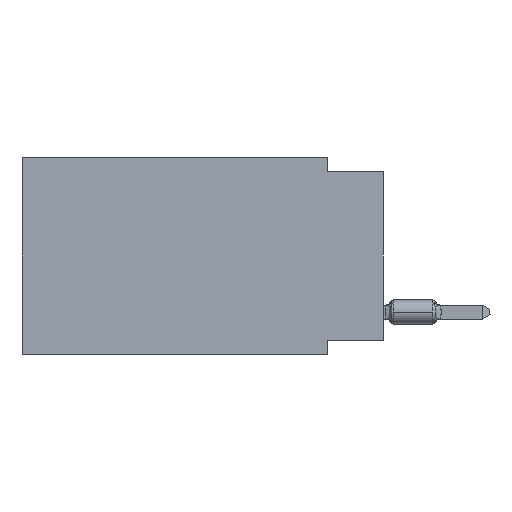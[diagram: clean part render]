
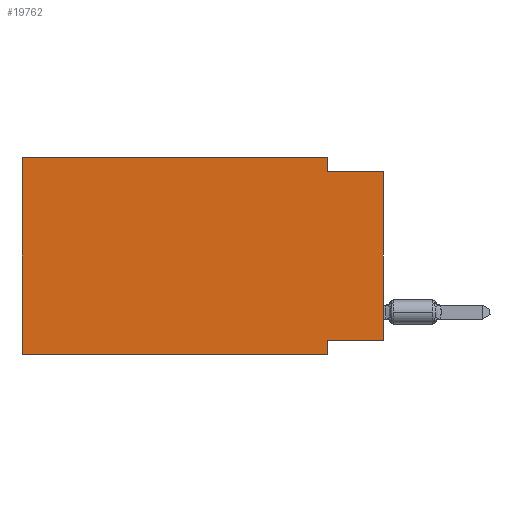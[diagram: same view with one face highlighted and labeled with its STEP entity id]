
A CAD part, left-side view. The second image highlights one B-rep face of the part: STEP entity #19762.
In plain terms, the highlighted planar face has unit normal (-1, 0, 0).
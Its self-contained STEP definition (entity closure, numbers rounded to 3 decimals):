
#37 = EDGE_CURVE ( 'NONE', #6962, #99822, #56680, .T. ) ;
#1829 = EDGE_CURVE ( 'NONE', #4040, #88119, #16245, .T. ) ;
#4040 = VERTEX_POINT ( 'NONE', #28221 ) ;
#5205 = CARTESIAN_POINT ( 'NONE',  ( 0., 0., -0.635 ) ) ;
#6962 = VERTEX_POINT ( 'NONE', #52230 ) ;
#16245 = LINE ( 'NONE', #67094, #36881 ) ;
#16502 = ORIENTED_EDGE ( 'NONE', *, *, #37, .F. ) ;
#18574 = VECTOR ( 'NONE', #83175, 1000. ) ;
#18762 = CARTESIAN_POINT ( 'NONE',  ( 0., 16.383, 0. ) ) ;
#19762 = ADVANCED_FACE ( 'NONE', ( #98889 ), #105676, .F. ) ;
#21310 = VECTOR ( 'NONE', #98407, 1000. ) ;
#28221 = CARTESIAN_POINT ( 'NONE',  ( 0., 16.383, -8.89 ) ) ;
#31546 = AXIS2_PLACEMENT_3D ( 'NONE', #55934, #38963, #63288 ) ;
#32537 = LINE ( 'NONE', #107725, #70098 ) ;
#34352 = CARTESIAN_POINT ( 'NONE',  ( 0., 0., -0.635 ) ) ;
#35883 = CARTESIAN_POINT ( 'NONE',  ( 0., 16.383, 0. ) ) ;
#36881 = VECTOR ( 'NONE', #58614, 1000. ) ;
#37529 = CARTESIAN_POINT ( 'NONE',  ( 0., 0., -8.255 ) ) ;
#38066 = EDGE_LOOP ( 'NONE', ( #58381, #95576, #74974, #60389, #82008, #105151, #45920, #16502 ) ) ;
#38711 = EDGE_CURVE ( 'NONE', #99822, #88119, #32537, .T. ) ;
#38963 = DIRECTION ( 'NONE',  ( 1., 0., 0. ) ) ;
#45920 = ORIENTED_EDGE ( 'NONE', *, *, #38711, .F. ) ;
#47256 = VECTOR ( 'NONE', #78206, 1000. ) ;
#47416 = EDGE_CURVE ( 'NONE', #100924, #77672, #78816, .T. ) ;
#48139 = VERTEX_POINT ( 'NONE', #34352 ) ;
#52230 = CARTESIAN_POINT ( 'NONE',  ( 0., 0., -8.255 ) ) ;
#52786 = CARTESIAN_POINT ( 'NONE',  ( 0., 2.54, 0. ) ) ;
#53641 = CARTESIAN_POINT ( 'NONE',  ( 0., 2.54, -8.89 ) ) ;
#55934 = CARTESIAN_POINT ( 'NONE',  ( 0., 16.383, 0. ) ) ;
#56680 = LINE ( 'NONE', #37529, #88743 ) ;
#58381 = ORIENTED_EDGE ( 'NONE', *, *, #100848, .T. ) ;
#58614 = DIRECTION ( 'NONE',  ( 0., -1., 0. ) ) ;
#58934 = CARTESIAN_POINT ( 'NONE',  ( 0., 0., 0. ) ) ;
#60389 = ORIENTED_EDGE ( 'NONE', *, *, #47416, .F. ) ;
#63288 = DIRECTION ( 'NONE',  ( 0., 0., -1. ) ) ;
#63459 = VECTOR ( 'NONE', #92849, 1000. ) ;
#67094 = CARTESIAN_POINT ( 'NONE',  ( 0., 16.383, -8.89 ) ) ;
#68163 = CARTESIAN_POINT ( 'NONE',  ( 0., 2.54, 0. ) ) ;
#70098 = VECTOR ( 'NONE', #91898, 1000. ) ;
#73494 = CARTESIAN_POINT ( 'NONE',  ( 0., 2.54, -0.635 ) ) ;
#73655 = DIRECTION ( 'NONE',  ( 0., 1., 0. ) ) ;
#74141 = LINE ( 'NONE', #5205, #18574 ) ;
#74974 = ORIENTED_EDGE ( 'NONE', *, *, #99426, .F. ) ;
#77672 = VERTEX_POINT ( 'NONE', #68163 ) ;
#78206 = DIRECTION ( 'NONE',  ( 0., 0., -1. ) ) ;
#78816 = LINE ( 'NONE', #35883, #100861 ) ;
#82008 = ORIENTED_EDGE ( 'NONE', *, *, #94999, .F. ) ;
#82711 = LINE ( 'NONE', #58934, #63459 ) ;
#83175 = DIRECTION ( 'NONE',  ( 0., -1., 0. ) ) ;
#87913 = VERTEX_POINT ( 'NONE', #73494 ) ;
#88119 = VERTEX_POINT ( 'NONE', #53641 ) ;
#88265 = CARTESIAN_POINT ( 'NONE',  ( 0., 2.54, -8.255 ) ) ;
#88743 = VECTOR ( 'NONE', #73655, 1000. ) ;
#91898 = DIRECTION ( 'NONE',  ( 0., 0., -1. ) ) ;
#92849 = DIRECTION ( 'NONE',  ( 0., 0., 1. ) ) ;
#94999 = EDGE_CURVE ( 'NONE', #4040, #100924, #96190, .T. ) ;
#95576 = ORIENTED_EDGE ( 'NONE', *, *, #108126, .F. ) ;
#96190 = LINE ( 'NONE', #18762, #21310 ) ;
#96304 = LINE ( 'NONE', #52786, #47256 ) ;
#98407 = DIRECTION ( 'NONE',  ( 0., 0., 1. ) ) ;
#98889 = FACE_OUTER_BOUND ( 'NONE', #38066, .T. ) ;
#99426 = EDGE_CURVE ( 'NONE', #77672, #87913, #96304, .T. ) ;
#99822 = VERTEX_POINT ( 'NONE', #88265 ) ;
#100848 = EDGE_CURVE ( 'NONE', #6962, #48139, #82711, .T. ) ;
#100861 = VECTOR ( 'NONE', #104805, 1000. ) ;
#100924 = VERTEX_POINT ( 'NONE', #109237 ) ;
#104805 = DIRECTION ( 'NONE',  ( 0., -1., 0. ) ) ;
#105151 = ORIENTED_EDGE ( 'NONE', *, *, #1829, .T. ) ;
#105676 = PLANE ( 'NONE',  #31546 ) ;
#107725 = CARTESIAN_POINT ( 'NONE',  ( 0., 2.54, -8.89 ) ) ;
#108126 = EDGE_CURVE ( 'NONE', #87913, #48139, #74141, .T. ) ;
#109237 = CARTESIAN_POINT ( 'NONE',  ( 0., 16.383, 0. ) ) ;
